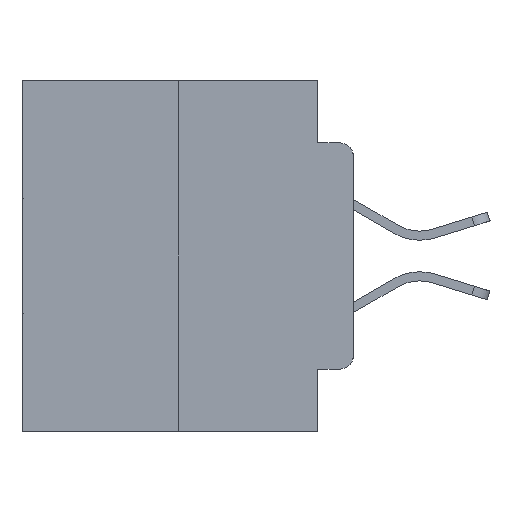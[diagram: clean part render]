
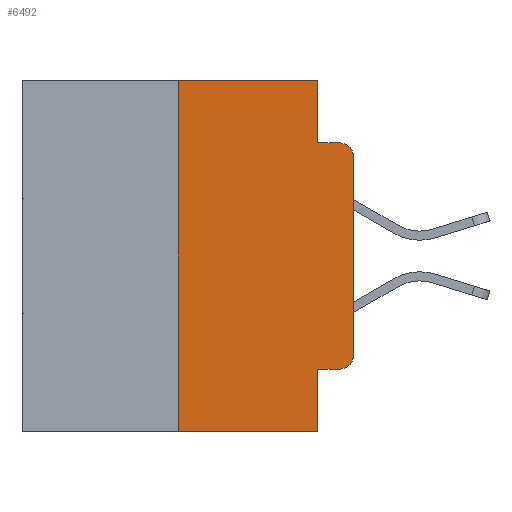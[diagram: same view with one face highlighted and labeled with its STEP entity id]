
A CAD part, left-side view. The second image highlights one B-rep face of the part: STEP entity #6492.
In plain terms, the highlighted planar face has unit normal (-1, 0, 0).
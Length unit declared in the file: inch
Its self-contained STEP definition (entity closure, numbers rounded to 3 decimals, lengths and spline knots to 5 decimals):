
#139 = ORIENTED_EDGE ( 'NONE', *, *, #20683, .F. ) ;
#418 = ORIENTED_EDGE ( 'NONE', *, *, #15304, .F. ) ;
#718 = ORIENTED_EDGE ( 'NONE', *, *, #11398, .T. ) ;
#777 = CARTESIAN_POINT ( 'NONE',  ( 0., 0., -0.3915 ) ) ;
#985 = DIRECTION ( 'NONE',  ( 0., 0., 1. ) ) ;
#1033 = ORIENTED_EDGE ( 'NONE', *, *, #19530, .F. ) ;
#1175 = EDGE_CURVE ( 'NONE', #5402, #10344, #12346, .T. ) ;
#1547 = EDGE_CURVE ( 'NONE', #18615, #1809, #15712, .T. ) ;
#1629 = ORIENTED_EDGE ( 'NONE', *, *, #25161, .T. ) ;
#1809 = VERTEX_POINT ( 'NONE', #4752 ) ;
#1893 = ORIENTED_EDGE ( 'NONE', *, *, #1175, .T. ) ;
#2169 = AXIS2_PLACEMENT_3D ( 'NONE', #16435, #2668, #11692 ) ;
#2668 = DIRECTION ( 'NONE',  ( -1., 0., 0. ) ) ;
#3360 = VECTOR ( 'NONE', #27542, 39.37008 ) ;
#4296 = VERTEX_POINT ( 'NONE', #8901 ) ;
#4752 = CARTESIAN_POINT ( 'NONE',  ( 0., 0.02, -0.0885 ) ) ;
#4799 = CARTESIAN_POINT ( 'NONE',  ( 0., 0.051, 0. ) ) ;
#5069 = FACE_OUTER_BOUND ( 'NONE', #6498, .T. ) ;
#5177 = DIRECTION ( 'NONE',  ( 0., 0., -1. ) ) ;
#5402 = VERTEX_POINT ( 'NONE', #14962 ) ;
#6143 = VECTOR ( 'NONE', #22459, 39.37008 ) ;
#6273 = CARTESIAN_POINT ( 'NONE',  ( 0., 0.051, -0.0885 ) ) ;
#6492 = ADVANCED_FACE ( 'NONE', ( #5069 ), #14021, .F. ) ;
#6498 = EDGE_LOOP ( 'NONE', ( #10968, #10338, #9689, #9294, #139, #418, #718, #1033, #1629, #1893 ) ) ;
#7400 = VERTEX_POINT ( 'NONE', #4799 ) ;
#8347 = LINE ( 'NONE', #16624, #24731 ) ;
#8901 = CARTESIAN_POINT ( 'NONE',  ( 0., 0.25, 0. ) ) ;
#9069 = DIRECTION ( 'NONE',  ( 0., -1., 0. ) ) ;
#9213 = EDGE_CURVE ( 'NONE', #15138, #1809, #10601, .T. ) ;
#9294 = ORIENTED_EDGE ( 'NONE', *, *, #13828, .F. ) ;
#9363 = DIRECTION ( 'NONE',  ( -1., 0., 0. ) ) ;
#9539 = CARTESIAN_POINT ( 'NONE',  ( 0., 0.473, 0. ) ) ;
#9689 = ORIENTED_EDGE ( 'NONE', *, *, #1547, .F. ) ;
#10338 = ORIENTED_EDGE ( 'NONE', *, *, #9213, .T. ) ;
#10344 = VERTEX_POINT ( 'NONE', #777 ) ;
#10566 = VERTEX_POINT ( 'NONE', #14983 ) ;
#10601 = CIRCLE ( 'NONE', #18489, 0.02 ) ;
#10724 = EDGE_CURVE ( 'NONE', #10344, #15138, #24157, .T. ) ;
#10827 = LINE ( 'NONE', #21225, #3360 ) ;
#10968 = ORIENTED_EDGE ( 'NONE', *, *, #10724, .T. ) ;
#11398 = EDGE_CURVE ( 'NONE', #10566, #25339, #24164, .T. ) ;
#11427 = CARTESIAN_POINT ( 'NONE',  ( 0., 0.051, 0. ) ) ;
#11692 = DIRECTION ( 'NONE',  ( 0., 0., -1. ) ) ;
#12346 = CIRCLE ( 'NONE', #2169, 0.02 ) ;
#12899 = VECTOR ( 'NONE', #9069, 39.37008 ) ;
#12985 = DIRECTION ( 'NONE',  ( 0., -1., 0. ) ) ;
#13243 = CARTESIAN_POINT ( 'NONE',  ( 0., 0., 0. ) ) ;
#13260 = AXIS2_PLACEMENT_3D ( 'NONE', #9539, #18305, #5177 ) ;
#13565 = VECTOR ( 'NONE', #17542, 39.37008 ) ;
#13594 = VECTOR ( 'NONE', #20402, 39.37008 ) ;
#13763 = VECTOR ( 'NONE', #26246, 39.37008 ) ;
#13828 = EDGE_CURVE ( 'NONE', #7400, #18615, #18760, .T. ) ;
#14021 = PLANE ( 'NONE',  #13260 ) ;
#14133 = CARTESIAN_POINT ( 'NONE',  ( 0., 0.051, -0.0885 ) ) ;
#14279 = LINE ( 'NONE', #26720, #13594 ) ;
#14962 = CARTESIAN_POINT ( 'NONE',  ( 0., 0.02, -0.4115 ) ) ;
#14983 = CARTESIAN_POINT ( 'NONE',  ( 0., 0.25, -0.5 ) ) ;
#15138 = VERTEX_POINT ( 'NONE', #22456 ) ;
#15304 = EDGE_CURVE ( 'NONE', #10566, #4296, #8347, .T. ) ;
#15659 = CARTESIAN_POINT ( 'NONE',  ( 0., 0.051, -0.4115 ) ) ;
#15712 = LINE ( 'NONE', #6273, #26224 ) ;
#16435 = CARTESIAN_POINT ( 'NONE',  ( 0., 0.02, -0.3915 ) ) ;
#16624 = CARTESIAN_POINT ( 'NONE',  ( 0., 0.25, 0. ) ) ;
#17542 = DIRECTION ( 'NONE',  ( 0., 0., 1. ) ) ;
#18199 = CARTESIAN_POINT ( 'NONE',  ( 0., 0.473, 0. ) ) ;
#18305 = DIRECTION ( 'NONE',  ( 1., 0., 0. ) ) ;
#18418 = VERTEX_POINT ( 'NONE', #15659 ) ;
#18489 = AXIS2_PLACEMENT_3D ( 'NONE', #22222, #9363, #24298 ) ;
#18615 = VERTEX_POINT ( 'NONE', #14133 ) ;
#18760 = LINE ( 'NONE', #11427, #13763 ) ;
#19530 = EDGE_CURVE ( 'NONE', #18418, #25339, #14279, .T. ) ;
#19802 = CARTESIAN_POINT ( 'NONE',  ( 0., 0.473, -0.5 ) ) ;
#20402 = DIRECTION ( 'NONE',  ( 0., 0., -1. ) ) ;
#20683 = EDGE_CURVE ( 'NONE', #4296, #7400, #23382, .T. ) ;
#21225 = CARTESIAN_POINT ( 'NONE',  ( 0., 0.051, -0.4115 ) ) ;
#22222 = CARTESIAN_POINT ( 'NONE',  ( 0., 0.02, -0.1085 ) ) ;
#22456 = CARTESIAN_POINT ( 'NONE',  ( 0., 0., -0.1085 ) ) ;
#22459 = DIRECTION ( 'NONE',  ( 0., -1., 0. ) ) ;
#23382 = LINE ( 'NONE', #18199, #6143 ) ;
#24157 = LINE ( 'NONE', #13243, #13565 ) ;
#24164 = LINE ( 'NONE', #19802, #12899 ) ;
#24298 = DIRECTION ( 'NONE',  ( 0., 0., -1. ) ) ;
#24731 = VECTOR ( 'NONE', #985, 39.37008 ) ;
#25161 = EDGE_CURVE ( 'NONE', #18418, #5402, #10827, .T. ) ;
#25339 = VERTEX_POINT ( 'NONE', #27987 ) ;
#26224 = VECTOR ( 'NONE', #12985, 39.37008 ) ;
#26246 = DIRECTION ( 'NONE',  ( 0., 0., -1. ) ) ;
#26720 = CARTESIAN_POINT ( 'NONE',  ( 0., 0.051, 0. ) ) ;
#27542 = DIRECTION ( 'NONE',  ( 0., -1., 0. ) ) ;
#27987 = CARTESIAN_POINT ( 'NONE',  ( 0., 0.051, -0.5 ) ) ;
